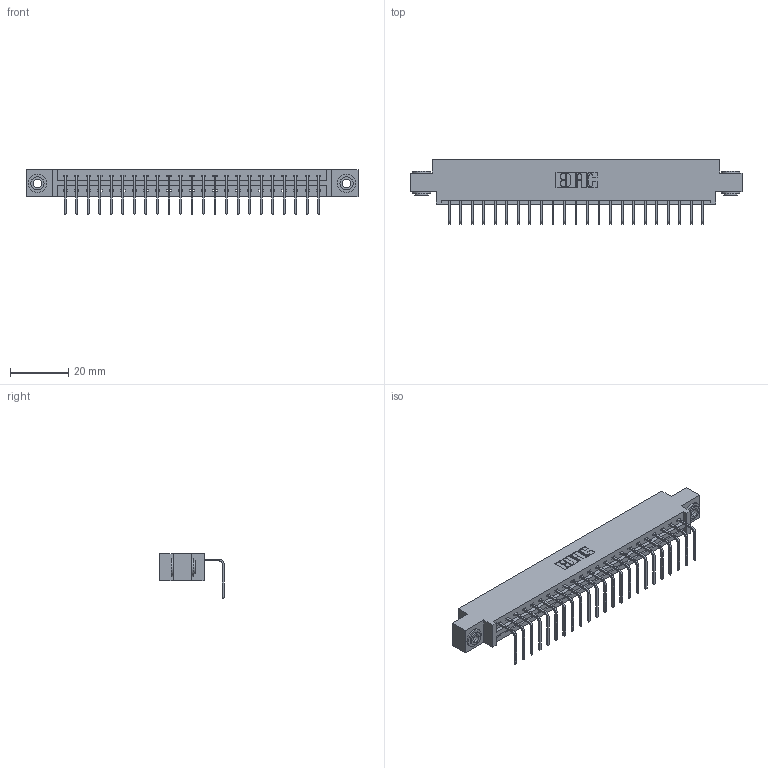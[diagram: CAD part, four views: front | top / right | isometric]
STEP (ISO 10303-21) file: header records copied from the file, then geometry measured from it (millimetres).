
FILE_DESCRIPTION (( 'STEP AP203' ), '1' );
FILE_NAME ('337-023-558-603.STEP', '2018-08-05T17:40:39', ( '' ), ( '' ), 'SwSTEP 2.0', 'SolidWorks 2016', '' );
FILE_SCHEMA (( 'CONFIG_CONTROL_DESIGN' ));
Length unit declared in the file: inch
Products named in the file (4): 337 Part_0.170 Offset - 0.156 Dia-TH; 345-292-001_558 Tail - 2; 345-250-002_345-250-002-102; 337-023-558-603
Assembly tree (26 placements, depth 2):
  337-023-558-603
    337 Part_0.170 Offset - 0.156 Dia-TH
    345-292-001_558 Tail - 2  x23
    345-250-002_345-250-002-102  x2
Bounding box: 114.15 x 22.17 x 15.37 mm (x, y, z)
Volume: 11604.5 mm3; surface area: 12686 mm2
Topology: 26 solids, 26 shells, 1628 faces, 4861 edges, 3206 vertices
Faces by surface type: plane 1188, cylinder 432, cone 8
Entity records: 20420 total; most frequent: CARTESIAN_POINT 3534, ORIENTED_EDGE 3486, DIRECTION 3047, EDGE_CURVE 1743, VECTOR 1591, LINE 1591, VERTEX_POINT 1158, AXIS2_PLACEMENT_3D 728
